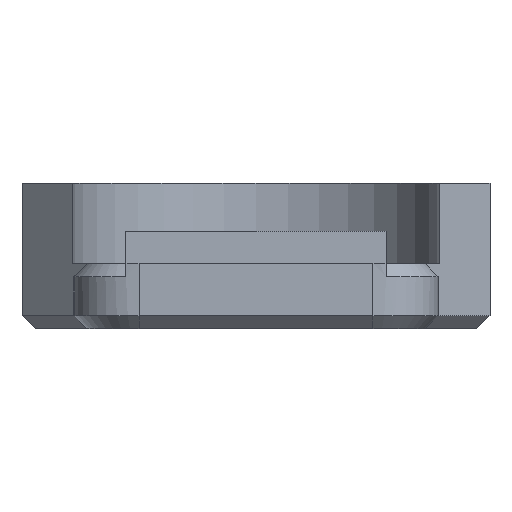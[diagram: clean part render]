
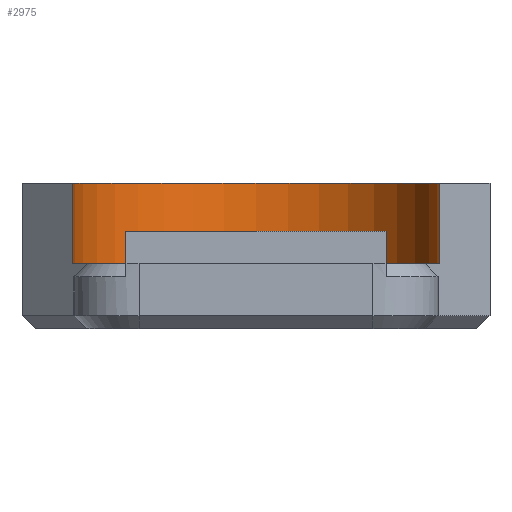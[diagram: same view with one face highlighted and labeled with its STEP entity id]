
A CAD part, front view. The second image highlights one B-rep face of the part: STEP entity #2975.
In plain terms, the highlighted cylindrical face has radius 8.985 mm (diameter 17.97 mm), a partial arc.
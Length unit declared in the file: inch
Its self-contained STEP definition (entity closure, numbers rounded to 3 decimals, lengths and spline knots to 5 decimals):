
#308 = CARTESIAN_POINT ( 'NONE',  ( 0.35375, 0., 0.27928 ) ) ;
#312 = VERTEX_POINT ( 'NONE', #1487 ) ;
#634 = CARTESIAN_POINT ( 'NONE',  ( 0.35375, 0., 0.125 ) ) ;
#858 = ORIENTED_EDGE ( 'NONE', *, *, #2811, .F. ) ;
#1229 = DIRECTION ( 'NONE',  ( 0., 0., -1. ) ) ;
#1487 = CARTESIAN_POINT ( 'NONE',  ( -0.35375, 0., 0.125 ) ) ;
#1570 = EDGE_CURVE ( 'NONE', #2505, #312, #3095, .T. ) ;
#2305 = ORIENTED_EDGE ( 'NONE', *, *, #4626, .F. ) ;
#2505 = VERTEX_POINT ( 'NONE', #2620 ) ;
#2509 = CARTESIAN_POINT ( 'NONE',  ( 0., 0., 0.27928 ) ) ;
#2620 = CARTESIAN_POINT ( 'NONE',  ( -0.35375, 0., 0.27928 ) ) ;
#2811 = EDGE_CURVE ( 'NONE', #8576, #9372, #9922, .T. ) ;
#2975 = ADVANCED_FACE ( 'NONE', ( #11732 ), #12415, .F. ) ;
#3006 = EDGE_LOOP ( 'NONE', ( #13149, #858, #2305, #4604 ) ) ;
#3095 = LINE ( 'NONE', #10097, #11117 ) ;
#3822 = DIRECTION ( 'NONE',  ( 0., 0., -1. ) ) ;
#4089 = CIRCLE ( 'NONE', #7304, 0.35375 ) ;
#4604 = ORIENTED_EDGE ( 'NONE', *, *, #1570, .T. ) ;
#4626 = EDGE_CURVE ( 'NONE', #2505, #8576, #6107, .T. ) ;
#5150 = CARTESIAN_POINT ( 'NONE',  ( 0., 0., 0.27928 ) ) ;
#5719 = DIRECTION ( 'NONE',  ( -1., 0., 0. ) ) ;
#5984 = VECTOR ( 'NONE', #1229, 39.37008 ) ;
#6107 = CIRCLE ( 'NONE', #13099, 0.35375 ) ;
#6687 = DIRECTION ( 'NONE',  ( 0., 0., -1. ) ) ;
#7304 = AXIS2_PLACEMENT_3D ( 'NONE', #10939, #10896, #7751 ) ;
#7751 = DIRECTION ( 'NONE',  ( -1., 0., 0. ) ) ;
#8576 = VERTEX_POINT ( 'NONE', #8828 ) ;
#8828 = CARTESIAN_POINT ( 'NONE',  ( 0.35375, 0., 0.27928 ) ) ;
#9372 = VERTEX_POINT ( 'NONE', #634 ) ;
#9922 = LINE ( 'NONE', #308, #5984 ) ;
#10097 = CARTESIAN_POINT ( 'NONE',  ( -0.35375, 0., 0.27928 ) ) ;
#10889 = AXIS2_PLACEMENT_3D ( 'NONE', #2509, #6687, #5719 ) ;
#10896 = DIRECTION ( 'NONE',  ( 0., 0., -1. ) ) ;
#10939 = CARTESIAN_POINT ( 'NONE',  ( 0., 0., 0.125 ) ) ;
#11027 = EDGE_CURVE ( 'NONE', #312, #9372, #4089, .T. ) ;
#11117 = VECTOR ( 'NONE', #3822, 39.37008 ) ;
#11732 = FACE_OUTER_BOUND ( 'NONE', #3006, .T. ) ;
#12415 = CYLINDRICAL_SURFACE ( 'NONE', #10889, 0.35375 ) ;
#12461 = DIRECTION ( 'NONE',  ( 0., 0., -1. ) ) ;
#13099 = AXIS2_PLACEMENT_3D ( 'NONE', #5150, #12461, #13567 ) ;
#13149 = ORIENTED_EDGE ( 'NONE', *, *, #11027, .T. ) ;
#13567 = DIRECTION ( 'NONE',  ( -1., 0., 0. ) ) ;
